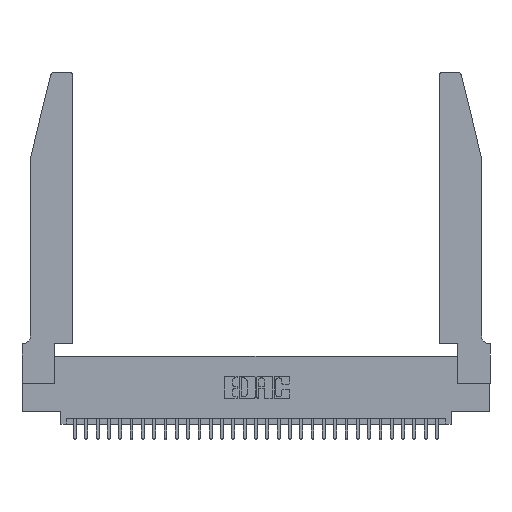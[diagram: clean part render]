
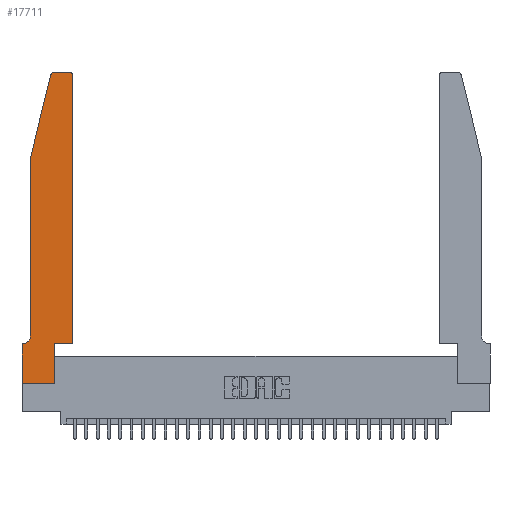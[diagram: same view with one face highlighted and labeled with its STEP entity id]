
A CAD part, top view. The second image highlights one B-rep face of the part: STEP entity #17711.
In plain terms, the highlighted planar face has unit normal (0, 0, 1).
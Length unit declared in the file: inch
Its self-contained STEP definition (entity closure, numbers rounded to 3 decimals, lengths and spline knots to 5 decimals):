
#687 = VERTEX_POINT ( 'NONE', #27326 ) ;
#877 = VECTOR ( 'NONE', #28938, 39.37008 ) ;
#1144 = DIRECTION ( 'NONE',  ( -1., 0., 0. ) ) ;
#2239 = LINE ( 'NONE', #21223, #21385 ) ;
#2408 = DIRECTION ( 'NONE',  ( 1., 0., 0. ) ) ;
#3049 = CIRCLE ( 'NONE', #21892, 0.03 ) ;
#3884 = DIRECTION ( 'NONE',  ( 0., 0., 1. ) ) ;
#4807 = EDGE_CURVE ( 'NONE', #11551, #4907, #3049, .T. ) ;
#4907 = VERTEX_POINT ( 'NONE', #20225 ) ;
#5005 = VERTEX_POINT ( 'NONE', #23477 ) ;
#5537 = AXIS2_PLACEMENT_3D ( 'NONE', #13184, #30342, #15713 ) ;
#5748 = EDGE_CURVE ( 'NONE', #20503, #28343, #2239, .T. ) ;
#6431 = CARTESIAN_POINT ( 'NONE',  ( 0.0055, 0.42, 0.37 ) ) ;
#6542 = LINE ( 'NONE', #20587, #17525 ) ;
#7200 = ORIENTED_EDGE ( 'NONE', *, *, #12295, .T. ) ;
#7723 = CARTESIAN_POINT ( 'NONE',  ( 0.2865, 0.35, 0.37 ) ) ;
#7824 = DIRECTION ( 'NONE',  ( -1., 0., 0. ) ) ;
#7905 = VERTEX_POINT ( 'NONE', #19820 ) ;
#7968 = CARTESIAN_POINT ( 'NONE',  ( 0., 0., 0.37 ) ) ;
#8134 = CIRCLE ( 'NONE', #9994, 0.07 ) ;
#8140 = DIRECTION ( 'NONE',  ( -0.239, -0.971, 0. ) ) ;
#8303 = LINE ( 'NONE', #23661, #14206 ) ;
#8916 = DIRECTION ( 'NONE',  ( 1., 0., 0. ) ) ;
#8974 = DIRECTION ( 'NONE',  ( -1., 0., 0. ) ) ;
#9163 = ORIENTED_EDGE ( 'NONE', *, *, #18334, .T. ) ;
#9713 = ORIENTED_EDGE ( 'NONE', *, *, #24212, .T. ) ;
#9994 = AXIS2_PLACEMENT_3D ( 'NONE', #6431, #23819, #8974 ) ;
#10183 = VERTEX_POINT ( 'NONE', #17752 ) ;
#10373 = LINE ( 'NONE', #28334, #16219 ) ;
#11551 = VERTEX_POINT ( 'NONE', #12518 ) ;
#12295 = EDGE_CURVE ( 'NONE', #28343, #28069, #12986, .T. ) ;
#12462 = VECTOR ( 'NONE', #1144, 39.37008 ) ;
#12518 = CARTESIAN_POINT ( 'NONE',  ( 0.4505, 2.72, 0.37 ) ) ;
#12645 = ORIENTED_EDGE ( 'NONE', *, *, #5748, .T. ) ;
#12897 = CARTESIAN_POINT ( 'NONE',  ( 0.0755, 0.35, 0.37 ) ) ;
#12986 = LINE ( 'NONE', #7723, #19587 ) ;
#13184 = CARTESIAN_POINT ( 'NONE',  ( 0.284, 2.72, 0.37 ) ) ;
#13938 = VERTEX_POINT ( 'NONE', #31669 ) ;
#14007 = LINE ( 'NONE', #16163, #12462 ) ;
#14017 = VECTOR ( 'NONE', #7824, 39.37008 ) ;
#14029 = ORIENTED_EDGE ( 'NONE', *, *, #26292, .T. ) ;
#14206 = VECTOR ( 'NONE', #26115, 39.37008 ) ;
#14840 = EDGE_CURVE ( 'NONE', #30222, #7905, #8134, .T. ) ;
#15236 = EDGE_LOOP ( 'NONE', ( #19075, #25948, #27665, #14029, #24770, #9713, #9163, #12645, #7200, #27803, #29139, #23417 ) ) ;
#15407 = EDGE_CURVE ( 'NONE', #4907, #5005, #14007, .T. ) ;
#15713 = DIRECTION ( 'NONE',  ( 1., 0., 0. ) ) ;
#16163 = CARTESIAN_POINT ( 'NONE',  ( 0.2605, 2.75, 0.37 ) ) ;
#16219 = VECTOR ( 'NONE', #30780, 39.37008 ) ;
#16412 = CARTESIAN_POINT ( 'NONE',  ( 0., 0.35, 0.37 ) ) ;
#17423 = DIRECTION ( 'NONE',  ( 0., 0., 1. ) ) ;
#17525 = VECTOR ( 'NONE', #8140, 39.37008 ) ;
#17711 = ADVANCED_FACE ( 'NONE', ( #26166 ), #31021, .T. ) ;
#17752 = CARTESIAN_POINT ( 'NONE',  ( 0.4505, 0.35, 0.37 ) ) ;
#18334 = EDGE_CURVE ( 'NONE', #687, #20503, #8303, .T. ) ;
#19075 = ORIENTED_EDGE ( 'NONE', *, *, #15407, .T. ) ;
#19214 = DIRECTION ( 'NONE',  ( 1., 0., 0. ) ) ;
#19240 = CARTESIAN_POINT ( 'NONE',  ( 0.4505, 0.35, 0.37 ) ) ;
#19587 = VECTOR ( 'NONE', #27508, 39.37008 ) ;
#19615 = EDGE_CURVE ( 'NONE', #28069, #10183, #24669, .T. ) ;
#19820 = CARTESIAN_POINT ( 'NONE',  ( 0.0055, 0.35, 0.37 ) ) ;
#20190 = EDGE_CURVE ( 'NONE', #10183, #11551, #27286, .T. ) ;
#20225 = CARTESIAN_POINT ( 'NONE',  ( 0.4205, 2.75, 0.37 ) ) ;
#20503 = VERTEX_POINT ( 'NONE', #7968 ) ;
#20587 = CARTESIAN_POINT ( 'NONE',  ( 0.0755, 2., 0.37 ) ) ;
#20703 = CARTESIAN_POINT ( 'NONE',  ( 0.2865, 0., 0.37 ) ) ;
#21223 = CARTESIAN_POINT ( 'NONE',  ( 0., 0., 0.37 ) ) ;
#21378 = DIRECTION ( 'NONE',  ( 1., 0., 0. ) ) ;
#21385 = VECTOR ( 'NONE', #8916, 39.37008 ) ;
#21892 = AXIS2_PLACEMENT_3D ( 'NONE', #30429, #17423, #2408 ) ;
#23417 = ORIENTED_EDGE ( 'NONE', *, *, #4807, .T. ) ;
#23477 = CARTESIAN_POINT ( 'NONE',  ( 0.284, 2.75, 0.37 ) ) ;
#23661 = CARTESIAN_POINT ( 'NONE',  ( 0., 0., 0.37 ) ) ;
#23819 = DIRECTION ( 'NONE',  ( 0., 0., -1. ) ) ;
#24010 = VERTEX_POINT ( 'NONE', #24541 ) ;
#24212 = EDGE_CURVE ( 'NONE', #7905, #687, #27093, .T. ) ;
#24286 = EDGE_CURVE ( 'NONE', #13938, #24010, #6542, .T. ) ;
#24541 = CARTESIAN_POINT ( 'NONE',  ( 0.0755, 2., 0.37 ) ) ;
#24669 = LINE ( 'NONE', #28799, #30351 ) ;
#24770 = ORIENTED_EDGE ( 'NONE', *, *, #14840, .T. ) ;
#25690 = CARTESIAN_POINT ( 'NONE',  ( 0.2865, 0.35, 0.37 ) ) ;
#25948 = ORIENTED_EDGE ( 'NONE', *, *, #28936, .T. ) ;
#26115 = DIRECTION ( 'NONE',  ( 0., -1., 0. ) ) ;
#26166 = FACE_OUTER_BOUND ( 'NONE', #15236, .T. ) ;
#26292 = EDGE_CURVE ( 'NONE', #24010, #30222, #10373, .T. ) ;
#27093 = LINE ( 'NONE', #12897, #14017 ) ;
#27163 = CIRCLE ( 'NONE', #5537, 0.03 ) ;
#27286 = LINE ( 'NONE', #19240, #877 ) ;
#27326 = CARTESIAN_POINT ( 'NONE',  ( 0., 0.35, 0.37 ) ) ;
#27508 = DIRECTION ( 'NONE',  ( 0., 1., 0. ) ) ;
#27665 = ORIENTED_EDGE ( 'NONE', *, *, #24286, .T. ) ;
#27803 = ORIENTED_EDGE ( 'NONE', *, *, #19615, .T. ) ;
#28069 = VERTEX_POINT ( 'NONE', #25690 ) ;
#28334 = CARTESIAN_POINT ( 'NONE',  ( 0.0755, 2., 0.37 ) ) ;
#28343 = VERTEX_POINT ( 'NONE', #20703 ) ;
#28799 = CARTESIAN_POINT ( 'NONE',  ( 0.4505, 0.35, 0.37 ) ) ;
#28936 = EDGE_CURVE ( 'NONE', #5005, #13938, #27163, .T. ) ;
#28938 = DIRECTION ( 'NONE',  ( 0., 1., 0. ) ) ;
#29139 = ORIENTED_EDGE ( 'NONE', *, *, #20190, .T. ) ;
#30222 = VERTEX_POINT ( 'NONE', #30901 ) ;
#30342 = DIRECTION ( 'NONE',  ( 0., 0., 1. ) ) ;
#30351 = VECTOR ( 'NONE', #19214, 39.37008 ) ;
#30429 = CARTESIAN_POINT ( 'NONE',  ( 0.4205, 2.72, 0.37 ) ) ;
#30780 = DIRECTION ( 'NONE',  ( 0., -1., 0. ) ) ;
#30901 = CARTESIAN_POINT ( 'NONE',  ( 0.0755, 0.42, 0.37 ) ) ;
#31021 = PLANE ( 'NONE',  #31457 ) ;
#31457 = AXIS2_PLACEMENT_3D ( 'NONE', #16412, #3884, #21378 ) ;
#31669 = CARTESIAN_POINT ( 'NONE',  ( 0.25487, 2.72718, 0.37 ) ) ;
